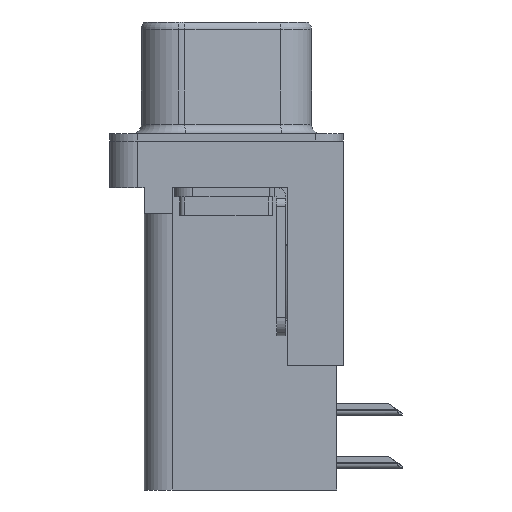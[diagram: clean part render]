
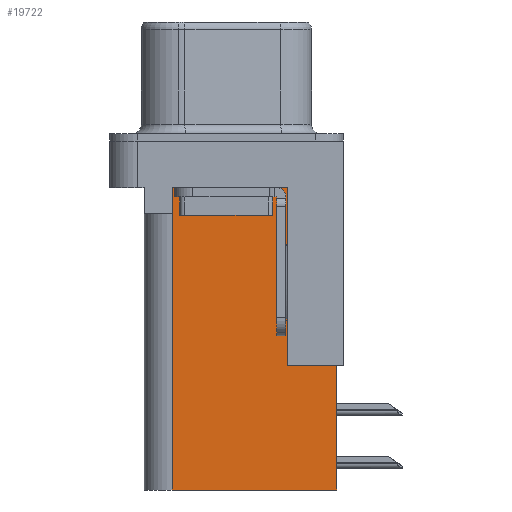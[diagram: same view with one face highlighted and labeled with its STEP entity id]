
A CAD part, left-side view. The second image highlights one B-rep face of the part: STEP entity #19722.
In plain terms, the highlighted planar face has unit normal (-1, 0, 0).
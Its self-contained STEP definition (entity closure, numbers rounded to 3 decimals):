
#986 = VECTOR ( 'NONE', #9994, 1000. ) ;
#1181 = VERTEX_POINT ( 'NONE', #21570 ) ;
#1302 = CARTESIAN_POINT ( 'NONE',  ( 3.7, -5.925, -18.76 ) ) ;
#1378 = DIRECTION ( 'NONE',  ( 0., 0., -1. ) ) ;
#1423 = CARTESIAN_POINT ( 'NONE',  ( 3.7, 2.895, -3.9 ) ) ;
#1862 = LINE ( 'NONE', #11551, #20148 ) ;
#1983 = DIRECTION ( 'NONE',  ( 0., 0., 1. ) ) ;
#2160 = EDGE_CURVE ( 'NONE', #9614, #4219, #5003, .T. ) ;
#2179 = VERTEX_POINT ( 'NONE', #1302 ) ;
#2731 = DIRECTION ( 'NONE',  ( 0., 0., -1. ) ) ;
#3168 = LINE ( 'NONE', #4445, #15779 ) ;
#3433 = VECTOR ( 'NONE', #1983, 1000. ) ;
#4157 = CARTESIAN_POINT ( 'NONE',  ( 3.7, -3.295, -18.76 ) ) ;
#4219 = VERTEX_POINT ( 'NONE', #5274 ) ;
#4445 = CARTESIAN_POINT ( 'NONE',  ( 3.7, -5.925, -2. ) ) ;
#4471 = LINE ( 'NONE', #6522, #986 ) ;
#4510 = ORIENTED_EDGE ( 'NONE', *, *, #19844, .F. ) ;
#5003 = LINE ( 'NONE', #1423, #9078 ) ;
#5030 = DIRECTION ( 'NONE',  ( 0., 1., 0. ) ) ;
#5088 = ORIENTED_EDGE ( 'NONE', *, *, #15538, .T. ) ;
#5274 = CARTESIAN_POINT ( 'NONE',  ( 3.7, 2.895, -3.9 ) ) ;
#5873 = DIRECTION ( 'NONE',  ( 1., 0., 0. ) ) ;
#5895 = VERTEX_POINT ( 'NONE', #7115 ) ;
#6522 = CARTESIAN_POINT ( 'NONE',  ( 3.7, -3.295, -2.5 ) ) ;
#7115 = CARTESIAN_POINT ( 'NONE',  ( 3.7, 2.925, -18.76 ) ) ;
#7515 = VERTEX_POINT ( 'NONE', #10300 ) ;
#7542 = VECTOR ( 'NONE', #20562, 1000. ) ;
#7624 = CARTESIAN_POINT ( 'NONE',  ( 3.7, 2.895, -2.5 ) ) ;
#7718 = VERTEX_POINT ( 'NONE', #17654 ) ;
#8519 = CARTESIAN_POINT ( 'NONE',  ( 3.7, 0., -3.9 ) ) ;
#9078 = VECTOR ( 'NONE', #1378, 1000. ) ;
#9614 = VERTEX_POINT ( 'NONE', #7624 ) ;
#9994 = DIRECTION ( 'NONE',  ( 0., 1., 0. ) ) ;
#10300 = CARTESIAN_POINT ( 'NONE',  ( 3.7, -3.295, -2.5 ) ) ;
#11551 = CARTESIAN_POINT ( 'NONE',  ( 3.7, -3.295, -18.76 ) ) ;
#11682 = VECTOR ( 'NONE', #18407, 1000. ) ;
#12043 = LINE ( 'NONE', #8519, #20622 ) ;
#12302 = CARTESIAN_POINT ( 'NONE',  ( 3.7, 2.925, -18.76 ) ) ;
#12681 = LINE ( 'NONE', #18838, #7542 ) ;
#12901 = EDGE_CURVE ( 'NONE', #5895, #1181, #21704, .T. ) ;
#13233 = DIRECTION ( 'NONE',  ( 0., 1., 0. ) ) ;
#13285 = ORIENTED_EDGE ( 'NONE', *, *, #13362, .T. ) ;
#13362 = EDGE_CURVE ( 'NONE', #7515, #9614, #4471, .T. ) ;
#13453 = EDGE_CURVE ( 'NONE', #4219, #1181, #12043, .T. ) ;
#14040 = EDGE_LOOP ( 'NONE', ( #13285, #21957, #16229, #20446, #20409, #4510, #5088, #20146 ) ) ;
#14624 = AXIS2_PLACEMENT_3D ( 'NONE', #4157, #5873, #17905 ) ;
#15538 = EDGE_CURVE ( 'NONE', #7718, #17344, #16197, .T. ) ;
#15779 = VECTOR ( 'NONE', #2731, 1000. ) ;
#16170 = PLANE ( 'NONE',  #14624 ) ;
#16197 = LINE ( 'NONE', #21807, #11682 ) ;
#16229 = ORIENTED_EDGE ( 'NONE', *, *, #13453, .T. ) ;
#16826 = EDGE_CURVE ( 'NONE', #17344, #7515, #12681, .T. ) ;
#17344 = VERTEX_POINT ( 'NONE', #21901 ) ;
#17654 = CARTESIAN_POINT ( 'NONE',  ( 3.7, -5.925, -12.05 ) ) ;
#17905 = DIRECTION ( 'NONE',  ( 0., 1., 0. ) ) ;
#17965 = EDGE_CURVE ( 'NONE', #2179, #5895, #1862, .T. ) ;
#18407 = DIRECTION ( 'NONE',  ( 0., 1., 0. ) ) ;
#18484 = FACE_OUTER_BOUND ( 'NONE', #14040, .T. ) ;
#18838 = CARTESIAN_POINT ( 'NONE',  ( 3.7, -3.295, -18.76 ) ) ;
#19722 = ADVANCED_FACE ( 'NONE', ( #18484 ), #16170, .F. ) ;
#19844 = EDGE_CURVE ( 'NONE', #7718, #2179, #3168, .T. ) ;
#20146 = ORIENTED_EDGE ( 'NONE', *, *, #16826, .T. ) ;
#20148 = VECTOR ( 'NONE', #13233, 1000. ) ;
#20409 = ORIENTED_EDGE ( 'NONE', *, *, #17965, .F. ) ;
#20446 = ORIENTED_EDGE ( 'NONE', *, *, #12901, .F. ) ;
#20562 = DIRECTION ( 'NONE',  ( 0., 0., 1. ) ) ;
#20622 = VECTOR ( 'NONE', #5030, 1000. ) ;
#21570 = CARTESIAN_POINT ( 'NONE',  ( 3.7, 2.925, -3.9 ) ) ;
#21704 = LINE ( 'NONE', #12302, #3433 ) ;
#21807 = CARTESIAN_POINT ( 'NONE',  ( 3.7, -6.295, -12.05 ) ) ;
#21901 = CARTESIAN_POINT ( 'NONE',  ( 3.7, -3.295, -12.05 ) ) ;
#21957 = ORIENTED_EDGE ( 'NONE', *, *, #2160, .T. ) ;
